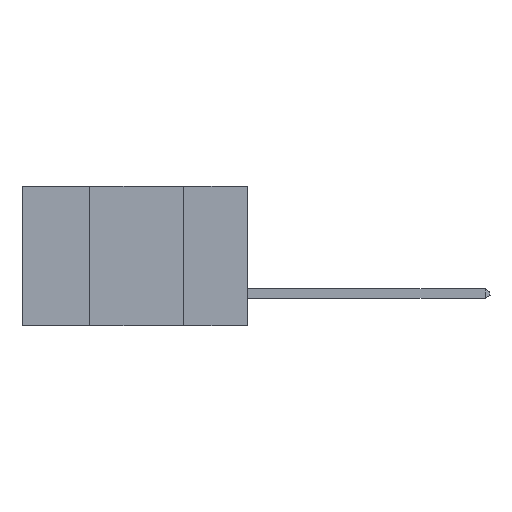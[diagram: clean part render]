
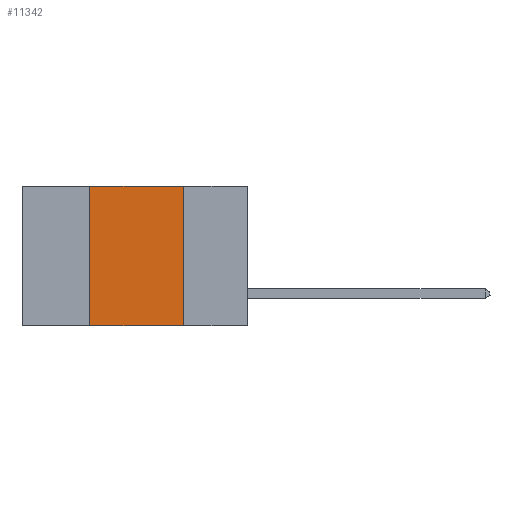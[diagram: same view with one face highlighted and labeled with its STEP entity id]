
A CAD part, left-side view. The second image highlights one B-rep face of the part: STEP entity #11342.
In plain terms, the highlighted planar face has unit normal (-1, 0, 0).
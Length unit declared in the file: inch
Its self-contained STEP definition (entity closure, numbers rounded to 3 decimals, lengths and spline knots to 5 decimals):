
#410 = ORIENTED_EDGE ( 'NONE', *, *, #9258, .F. ) ;
#669 = AXIS2_PLACEMENT_3D ( 'NONE', #6276, #1854, #11664 ) ;
#843 = DIRECTION ( 'NONE',  ( 0., 0., 1. ) ) ;
#862 = LINE ( 'NONE', #7660, #10366 ) ;
#976 = PLANE ( 'NONE',  #669 ) ;
#1854 = DIRECTION ( 'NONE',  ( 1., 0., 0. ) ) ;
#1952 = CARTESIAN_POINT ( 'NONE',  ( 0., 0.42, -0.37 ) ) ;
#2449 = EDGE_CURVE ( 'NONE', #7880, #11413, #8414, .T. ) ;
#2531 = VERTEX_POINT ( 'NONE', #10517 ) ;
#3212 = ORIENTED_EDGE ( 'NONE', *, *, #8957, .T. ) ;
#3611 = CARTESIAN_POINT ( 'NONE',  ( 0., 0.42, 0. ) ) ;
#4149 = EDGE_CURVE ( 'NONE', #11413, #9651, #6853, .T. ) ;
#4764 = DIRECTION ( 'NONE',  ( 0., 0., -1. ) ) ;
#4877 = ORIENTED_EDGE ( 'NONE', *, *, #4149, .F. ) ;
#5016 = ORIENTED_EDGE ( 'NONE', *, *, #2449, .F. ) ;
#5329 = DIRECTION ( 'NONE',  ( 0., -1., 0. ) ) ;
#5386 = CARTESIAN_POINT ( 'NONE',  ( 0., 0.42, 0. ) ) ;
#5641 = CARTESIAN_POINT ( 'NONE',  ( 0., 0.17, 0. ) ) ;
#6276 = CARTESIAN_POINT ( 'NONE',  ( 0., 0.6, 0. ) ) ;
#6661 = DIRECTION ( 'NONE',  ( 0., -1., 0. ) ) ;
#6673 = VECTOR ( 'NONE', #4764, 39.37008 ) ;
#6853 = LINE ( 'NONE', #10698, #11084 ) ;
#6880 = EDGE_LOOP ( 'NONE', ( #410, #4877, #5016, #3212 ) ) ;
#7440 = VECTOR ( 'NONE', #843, 39.37008 ) ;
#7660 = CARTESIAN_POINT ( 'NONE',  ( 0., 0.6, -0.37 ) ) ;
#7880 = VERTEX_POINT ( 'NONE', #1952 ) ;
#8414 = LINE ( 'NONE', #5386, #7440 ) ;
#8957 = EDGE_CURVE ( 'NONE', #7880, #2531, #862, .T. ) ;
#9258 = EDGE_CURVE ( 'NONE', #9651, #2531, #9365, .T. ) ;
#9365 = LINE ( 'NONE', #10213, #6673 ) ;
#9651 = VERTEX_POINT ( 'NONE', #5641 ) ;
#10213 = CARTESIAN_POINT ( 'NONE',  ( 0., 0.17, 0. ) ) ;
#10366 = VECTOR ( 'NONE', #6661, 39.37008 ) ;
#10517 = CARTESIAN_POINT ( 'NONE',  ( 0., 0.17, -0.37 ) ) ;
#10698 = CARTESIAN_POINT ( 'NONE',  ( 0., 0.6, 0. ) ) ;
#11084 = VECTOR ( 'NONE', #5329, 39.37008 ) ;
#11342 = ADVANCED_FACE ( 'NONE', ( #11676 ), #976, .F. ) ;
#11413 = VERTEX_POINT ( 'NONE', #3611 ) ;
#11664 = DIRECTION ( 'NONE',  ( 0., 0., -1. ) ) ;
#11676 = FACE_OUTER_BOUND ( 'NONE', #6880, .T. ) ;
